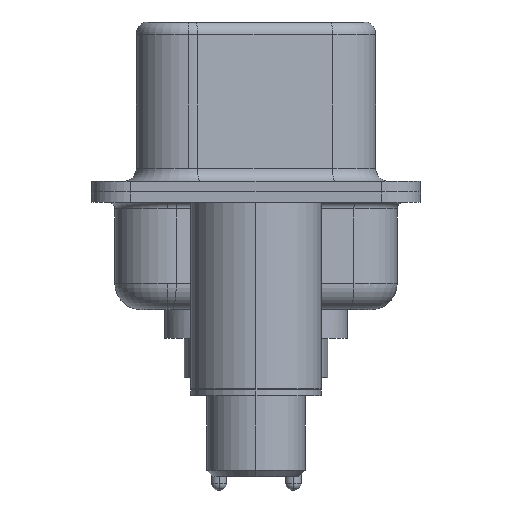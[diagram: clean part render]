
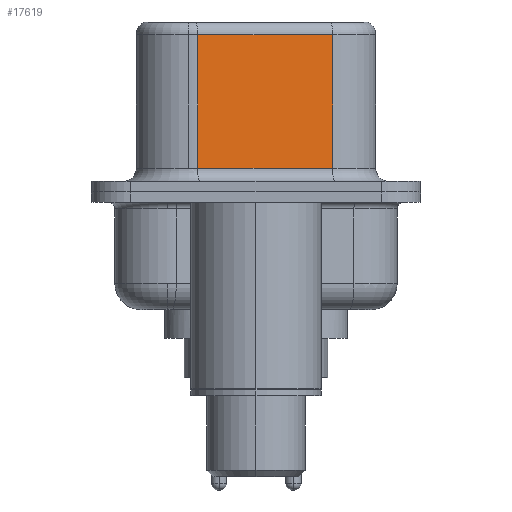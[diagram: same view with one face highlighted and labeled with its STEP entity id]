
A CAD part, left-side view. The second image highlights one B-rep face of the part: STEP entity #17619.
In plain terms, the highlighted planar face has unit normal (-0.985, -0.174, 0).
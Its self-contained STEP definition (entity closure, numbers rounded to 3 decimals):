
#137 = CARTESIAN_POINT ( 'NONE',  ( 4.565, -2.927, 6.02 ) ) ;
#643 = CARTESIAN_POINT ( 'NONE',  ( 4.565, -2.927, 6.02 ) ) ;
#1796 = VECTOR ( 'NONE', #16033, 1000. ) ;
#3195 = EDGE_LOOP ( 'NONE', ( #11950, #8408, #18165, #8524 ) ) ;
#3261 = VERTEX_POINT ( 'NONE', #9369 ) ;
#3760 = CARTESIAN_POINT ( 'NONE',  ( 4.565, -2.927, 6.52 ) ) ;
#4071 = PLANE ( 'NONE',  #19119 ) ;
#5345 = CARTESIAN_POINT ( 'NONE',  ( 3.655, 2.233, 6.02 ) ) ;
#5468 = FACE_OUTER_BOUND ( 'NONE', #3195, .T. ) ;
#5587 = DIRECTION ( 'NONE',  ( 0.985, 0.174, 0. ) ) ;
#5648 = VECTOR ( 'NONE', #6205, 1000. ) ;
#6205 = DIRECTION ( 'NONE',  ( 0., 0., -1. ) ) ;
#6272 = LINE ( 'NONE', #8225, #14482 ) ;
#6295 = LINE ( 'NONE', #3760, #1796 ) ;
#6703 = DIRECTION ( 'NONE',  ( 0.174, -0.985, 0. ) ) ;
#6714 = VERTEX_POINT ( 'NONE', #5345 ) ;
#6988 = EDGE_CURVE ( 'NONE', #19455, #3261, #6272, .T. ) ;
#7244 = LINE ( 'NONE', #643, #11296 ) ;
#7348 = CARTESIAN_POINT ( 'NONE',  ( 3.655, 2.233, 0.9 ) ) ;
#8225 = CARTESIAN_POINT ( 'NONE',  ( 4.565, -2.927, 0.9 ) ) ;
#8408 = ORIENTED_EDGE ( 'NONE', *, *, #14866, .T. ) ;
#8524 = ORIENTED_EDGE ( 'NONE', *, *, #6988, .T. ) ;
#8585 = CARTESIAN_POINT ( 'NONE',  ( 4.565, -2.927, 6.52 ) ) ;
#9369 = CARTESIAN_POINT ( 'NONE',  ( 4.565, -2.927, 0.9 ) ) ;
#10572 = EDGE_CURVE ( 'NONE', #6714, #19455, #10620, .T. ) ;
#10620 = LINE ( 'NONE', #15442, #5648 ) ;
#11296 = VECTOR ( 'NONE', #11328, 1000. ) ;
#11328 = DIRECTION ( 'NONE',  ( -0.174, 0.985, 0. ) ) ;
#11950 = ORIENTED_EDGE ( 'NONE', *, *, #12791, .F. ) ;
#12791 = EDGE_CURVE ( 'NONE', #17887, #3261, #6295, .T. ) ;
#14482 = VECTOR ( 'NONE', #6703, 1000. ) ;
#14866 = EDGE_CURVE ( 'NONE', #17887, #6714, #7244, .T. ) ;
#15442 = CARTESIAN_POINT ( 'NONE',  ( 3.655, 2.233, 6.52 ) ) ;
#16033 = DIRECTION ( 'NONE',  ( 0., 0., -1. ) ) ;
#16364 = DIRECTION ( 'NONE',  ( -0.174, 0.985, 0. ) ) ;
#17619 = ADVANCED_FACE ( 'NONE', ( #5468 ), #4071, .F. ) ;
#17887 = VERTEX_POINT ( 'NONE', #137 ) ;
#18165 = ORIENTED_EDGE ( 'NONE', *, *, #10572, .T. ) ;
#19119 = AXIS2_PLACEMENT_3D ( 'NONE', #8585, #5587, #16364 ) ;
#19455 = VERTEX_POINT ( 'NONE', #7348 ) ;
